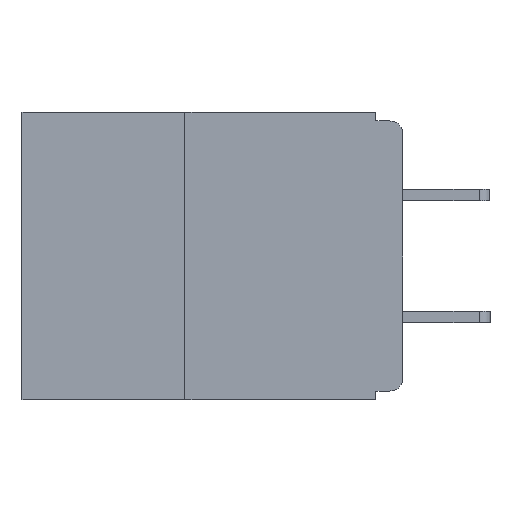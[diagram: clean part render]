
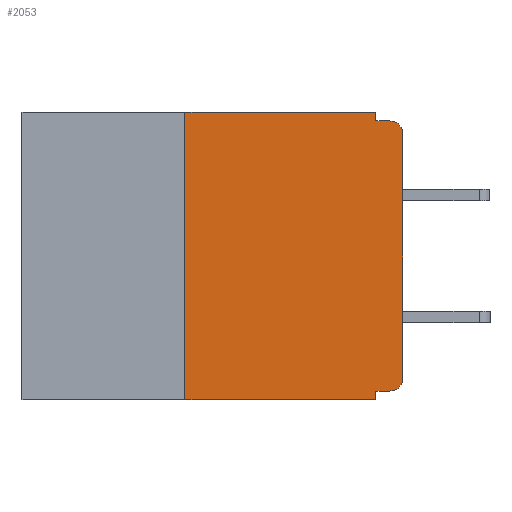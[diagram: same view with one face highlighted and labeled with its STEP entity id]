
A CAD part, left-side view. The second image highlights one B-rep face of the part: STEP entity #2053.
In plain terms, the highlighted planar face has unit normal (-1, 0, 0).
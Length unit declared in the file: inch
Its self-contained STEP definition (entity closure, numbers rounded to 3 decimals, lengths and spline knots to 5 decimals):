
#68 = ORIENTED_EDGE ( 'NONE', *, *, #4610, .F. ) ;
#137 = ORIENTED_EDGE ( 'NONE', *, *, #2863, .F. ) ;
#140 = CARTESIAN_POINT ( 'NONE',  ( 0., 0.031, -0.01 ) ) ;
#287 = ORIENTED_EDGE ( 'NONE', *, *, #6785, .T. ) ;
#533 = CIRCLE ( 'NONE', #3229, 0.015 ) ;
#849 = EDGE_CURVE ( 'NONE', #9049, #4069, #533, .T. ) ;
#934 = VERTEX_POINT ( 'NONE', #9615 ) ;
#1366 = ORIENTED_EDGE ( 'NONE', *, *, #6175, .F. ) ;
#1541 = VECTOR ( 'NONE', #2849, 39.37008 ) ;
#1547 = CARTESIAN_POINT ( 'NONE',  ( 0., 0.015, -0.025 ) ) ;
#1554 = VECTOR ( 'NONE', #4224, 39.37008 ) ;
#1664 = DIRECTION ( 'NONE',  ( 0., -1., 0. ) ) ;
#1665 = LINE ( 'NONE', #2850, #10718 ) ;
#1704 = CARTESIAN_POINT ( 'NONE',  ( 0., 0.25, -0.33 ) ) ;
#1788 = DIRECTION ( 'NONE',  ( 0., 0., -1. ) ) ;
#1818 = VECTOR ( 'NONE', #1664, 39.37008 ) ;
#1968 = DIRECTION ( 'NONE',  ( 0., 0., -1. ) ) ;
#1976 = EDGE_CURVE ( 'NONE', #5596, #7547, #7709, .T. ) ;
#2053 = ADVANCED_FACE ( 'NONE', ( #6623 ), #8391, .F. ) ;
#2101 = ORIENTED_EDGE ( 'NONE', *, *, #3678, .F. ) ;
#2111 = ORIENTED_EDGE ( 'NONE', *, *, #849, .T. ) ;
#2324 = DIRECTION ( 'NONE',  ( -1., 0., 0. ) ) ;
#2335 = CARTESIAN_POINT ( 'NONE',  ( 0., 0.015, -0.305 ) ) ;
#2654 = VECTOR ( 'NONE', #10750, 39.37008 ) ;
#2701 = DIRECTION ( 'NONE',  ( 0., 0., -1. ) ) ;
#2730 = LINE ( 'NONE', #9969, #5421 ) ;
#2849 = DIRECTION ( 'NONE',  ( 0., 0., 1. ) ) ;
#2850 = CARTESIAN_POINT ( 'NONE',  ( 0., 0.031, -0.33 ) ) ;
#2863 = EDGE_CURVE ( 'NONE', #10796, #934, #3654, .T. ) ;
#3088 = VERTEX_POINT ( 'NONE', #140 ) ;
#3190 = LINE ( 'NONE', #9120, #8055 ) ;
#3229 = AXIS2_PLACEMENT_3D ( 'NONE', #2335, #2324, #1788 ) ;
#3402 = VERTEX_POINT ( 'NONE', #10204 ) ;
#3586 = AXIS2_PLACEMENT_3D ( 'NONE', #9291, #9261, #7173 ) ;
#3600 = VERTEX_POINT ( 'NONE', #9990 ) ;
#3654 = LINE ( 'NONE', #1704, #1541 ) ;
#3678 = EDGE_CURVE ( 'NONE', #9049, #3600, #2730, .T. ) ;
#4069 = VERTEX_POINT ( 'NONE', #5429 ) ;
#4224 = DIRECTION ( 'NONE',  ( 0., -1., 0. ) ) ;
#4610 = EDGE_CURVE ( 'NONE', #934, #3402, #10868, .T. ) ;
#5294 = CARTESIAN_POINT ( 'NONE',  ( 0., 0.437, 0. ) ) ;
#5336 = DIRECTION ( 'NONE',  ( 0., 0., -1. ) ) ;
#5357 = DIRECTION ( 'NONE',  ( -1., 0., 0. ) ) ;
#5392 = CARTESIAN_POINT ( 'NONE',  ( 0., 0.031, -0.33 ) ) ;
#5421 = VECTOR ( 'NONE', #10041, 39.37008 ) ;
#5429 = CARTESIAN_POINT ( 'NONE',  ( 0., 0., -0.305 ) ) ;
#5436 = ORIENTED_EDGE ( 'NONE', *, *, #1976, .T. ) ;
#5596 = VERTEX_POINT ( 'NONE', #6633 ) ;
#5728 = ORIENTED_EDGE ( 'NONE', *, *, #7784, .T. ) ;
#6175 = EDGE_CURVE ( 'NONE', #3600, #7237, #1665, .T. ) ;
#6278 = DIRECTION ( 'NONE',  ( 0., 0., 1. ) ) ;
#6481 = ORIENTED_EDGE ( 'NONE', *, *, #6746, .F. ) ;
#6623 = FACE_OUTER_BOUND ( 'NONE', #8814, .T. ) ;
#6633 = CARTESIAN_POINT ( 'NONE',  ( 0., 0., -0.025 ) ) ;
#6719 = LINE ( 'NONE', #8031, #1818 ) ;
#6746 = EDGE_CURVE ( 'NONE', #3402, #3088, #3190, .T. ) ;
#6785 = EDGE_CURVE ( 'NONE', #10796, #7237, #9713, .T. ) ;
#7173 = DIRECTION ( 'NONE',  ( 0., 0., -1. ) ) ;
#7237 = VERTEX_POINT ( 'NONE', #5392 ) ;
#7547 = VERTEX_POINT ( 'NONE', #10128 ) ;
#7709 = CIRCLE ( 'NONE', #9238, 0.015 ) ;
#7784 = EDGE_CURVE ( 'NONE', #4069, #5596, #10546, .T. ) ;
#7864 = ORIENTED_EDGE ( 'NONE', *, *, #10885, .F. ) ;
#8031 = CARTESIAN_POINT ( 'NONE',  ( 0., 0., -0.01 ) ) ;
#8055 = VECTOR ( 'NONE', #1968, 39.37008 ) ;
#8391 = PLANE ( 'NONE',  #3586 ) ;
#8603 = CARTESIAN_POINT ( 'NONE',  ( 0., 0.015, -0.32 ) ) ;
#8814 = EDGE_LOOP ( 'NONE', ( #5728, #5436, #7864, #6481, #68, #137, #287, #1366, #2101, #2111 ) ) ;
#9049 = VERTEX_POINT ( 'NONE', #8603 ) ;
#9120 = CARTESIAN_POINT ( 'NONE',  ( 0., 0.031, 0. ) ) ;
#9238 = AXIS2_PLACEMENT_3D ( 'NONE', #1547, #5357, #5336 ) ;
#9261 = DIRECTION ( 'NONE',  ( 1., 0., 0. ) ) ;
#9291 = CARTESIAN_POINT ( 'NONE',  ( 0., 0.437, 0. ) ) ;
#9589 = CARTESIAN_POINT ( 'NONE',  ( 0., 0.25, -0.33 ) ) ;
#9615 = CARTESIAN_POINT ( 'NONE',  ( 0., 0.25, 0. ) ) ;
#9713 = LINE ( 'NONE', #9971, #2654 ) ;
#9969 = CARTESIAN_POINT ( 'NONE',  ( 0., 0., -0.32 ) ) ;
#9971 = CARTESIAN_POINT ( 'NONE',  ( 0., 0.437, -0.33 ) ) ;
#9990 = CARTESIAN_POINT ( 'NONE',  ( 0., 0.031, -0.32 ) ) ;
#10041 = DIRECTION ( 'NONE',  ( 0., 1., 0. ) ) ;
#10128 = CARTESIAN_POINT ( 'NONE',  ( 0., 0.015, -0.01 ) ) ;
#10204 = CARTESIAN_POINT ( 'NONE',  ( 0., 0.031, 0. ) ) ;
#10299 = VECTOR ( 'NONE', #6278, 39.37008 ) ;
#10446 = CARTESIAN_POINT ( 'NONE',  ( 0., 0., 0. ) ) ;
#10546 = LINE ( 'NONE', #10446, #10299 ) ;
#10718 = VECTOR ( 'NONE', #2701, 39.37008 ) ;
#10750 = DIRECTION ( 'NONE',  ( 0., -1., 0. ) ) ;
#10796 = VERTEX_POINT ( 'NONE', #9589 ) ;
#10868 = LINE ( 'NONE', #5294, #1554 ) ;
#10885 = EDGE_CURVE ( 'NONE', #3088, #7547, #6719, .T. ) ;
